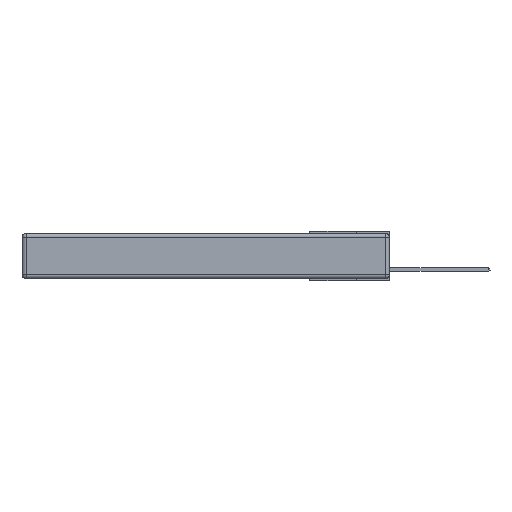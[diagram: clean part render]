
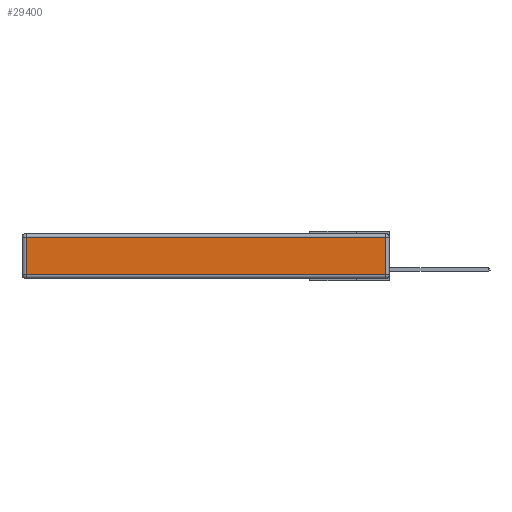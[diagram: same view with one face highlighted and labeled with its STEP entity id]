
A CAD part, left-side view. The second image highlights one B-rep face of the part: STEP entity #29400.
In plain terms, the highlighted planar face has unit normal (-1, 0, 0).
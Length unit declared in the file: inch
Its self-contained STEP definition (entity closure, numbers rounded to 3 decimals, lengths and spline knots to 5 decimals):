
#307 = CARTESIAN_POINT ( 'NONE',  ( 0., 0.03, -0.313 ) ) ;
#409 = EDGE_CURVE ( 'NONE', #13056, #21597, #27996, .T. ) ;
#420 = ORIENTED_EDGE ( 'NONE', *, *, #15917, .T. ) ;
#2072 = DIRECTION ( 'NONE',  ( 0., 0., -1. ) ) ;
#2676 = CARTESIAN_POINT ( 'NONE',  ( 0., 0., -0.343 ) ) ;
#2804 = CARTESIAN_POINT ( 'NONE',  ( 0., 0.03, -0.03 ) ) ;
#3037 = ORIENTED_EDGE ( 'NONE', *, *, #409, .T. ) ;
#6259 = DIRECTION ( 'NONE',  ( 0., 1., 0. ) ) ;
#6555 = LINE ( 'NONE', #7150, #18403 ) ;
#7021 = VECTOR ( 'NONE', #26757, 39.37008 ) ;
#7150 = CARTESIAN_POINT ( 'NONE',  ( 0., 2.72, -0.343 ) ) ;
#7268 = CARTESIAN_POINT ( 'NONE',  ( 0., 2.72, -0.03 ) ) ;
#8167 = EDGE_CURVE ( 'NONE', #19477, #30535, #30403, .T. ) ;
#8491 = CARTESIAN_POINT ( 'NONE',  ( 0., 2.75, -0.03 ) ) ;
#9570 = ORIENTED_EDGE ( 'NONE', *, *, #8167, .T. ) ;
#9812 = DIRECTION ( 'NONE',  ( 0., 0., 1. ) ) ;
#12013 = CARTESIAN_POINT ( 'NONE',  ( 0., 0.03, -0.343 ) ) ;
#12589 = DIRECTION ( 'NONE',  ( -1., 0., 0. ) ) ;
#13056 = VERTEX_POINT ( 'NONE', #29914 ) ;
#14167 = EDGE_CURVE ( 'NONE', #21597, #19477, #16959, .T. ) ;
#15835 = DIRECTION ( 'NONE',  ( 0., -1., 0. ) ) ;
#15868 = FACE_OUTER_BOUND ( 'NONE', #26712, .T. ) ;
#15917 = EDGE_CURVE ( 'NONE', #30535, #13056, #6555, .T. ) ;
#16915 = AXIS2_PLACEMENT_3D ( 'NONE', #2676, #12589, #9812 ) ;
#16959 = LINE ( 'NONE', #12013, #7021 ) ;
#18403 = VECTOR ( 'NONE', #2072, 39.37008 ) ;
#19477 = VERTEX_POINT ( 'NONE', #2804 ) ;
#20759 = VECTOR ( 'NONE', #15835, 39.37008 ) ;
#21597 = VERTEX_POINT ( 'NONE', #307 ) ;
#23312 = ORIENTED_EDGE ( 'NONE', *, *, #14167, .T. ) ;
#24481 = PLANE ( 'NONE',  #16915 ) ;
#26712 = EDGE_LOOP ( 'NONE', ( #3037, #23312, #9570, #420 ) ) ;
#26757 = DIRECTION ( 'NONE',  ( 0., 0., 1. ) ) ;
#27996 = LINE ( 'NONE', #28407, #20759 ) ;
#28407 = CARTESIAN_POINT ( 'NONE',  ( 0., 0., -0.313 ) ) ;
#29400 = ADVANCED_FACE ( 'NONE', ( #15868 ), #24481, .T. ) ;
#29658 = VECTOR ( 'NONE', #6259, 39.37008 ) ;
#29914 = CARTESIAN_POINT ( 'NONE',  ( 0., 2.72, -0.313 ) ) ;
#30403 = LINE ( 'NONE', #8491, #29658 ) ;
#30535 = VERTEX_POINT ( 'NONE', #7268 ) ;
